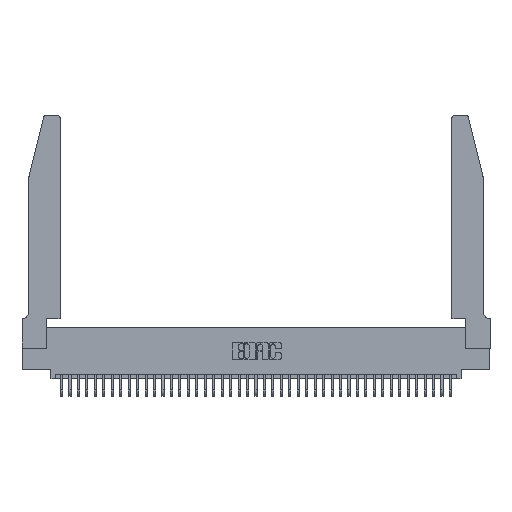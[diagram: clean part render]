
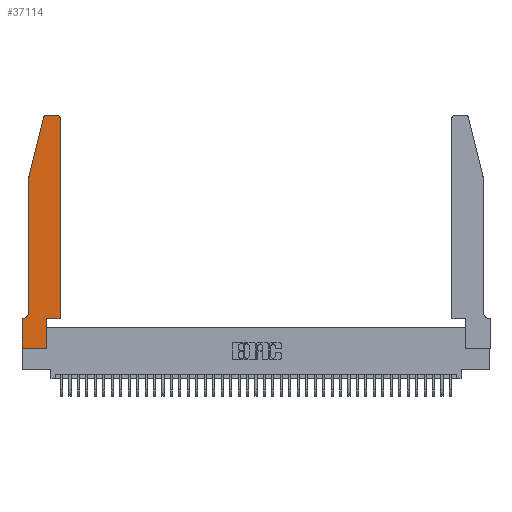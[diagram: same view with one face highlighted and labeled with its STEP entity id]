
A CAD part, top view. The second image highlights one B-rep face of the part: STEP entity #37114.
In plain terms, the highlighted planar face has unit normal (0, 0, 1).
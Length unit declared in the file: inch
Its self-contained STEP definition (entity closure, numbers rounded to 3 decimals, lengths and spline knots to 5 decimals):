
#99 = DIRECTION ( 'NONE',  ( 0., 0., -1. ) ) ;
#573 = VERTEX_POINT ( 'NONE', #23626 ) ;
#1099 = DIRECTION ( 'NONE',  ( -1., 0., 0. ) ) ;
#1113 = EDGE_CURVE ( 'NONE', #16538, #29028, #12907, .T. ) ;
#1559 = EDGE_CURVE ( 'NONE', #33392, #573, #23764, .T. ) ;
#1690 = VECTOR ( 'NONE', #23516, 39.37008 ) ;
#2515 = DIRECTION ( 'NONE',  ( 0., 1., 0. ) ) ;
#2747 = VERTEX_POINT ( 'NONE', #32198 ) ;
#3465 = EDGE_LOOP ( 'NONE', ( #12142, #10052, #17915, #38633, #32024, #14497, #37622, #26901, #16059, #22781, #12891, #10809 ) ) ;
#3533 = CARTESIAN_POINT ( 'NONE',  ( 0.2865, 0.35, 0.37 ) ) ;
#4565 = VECTOR ( 'NONE', #41761, 39.37008 ) ;
#4568 = DIRECTION ( 'NONE',  ( 0., 0., 1. ) ) ;
#5596 = AXIS2_PLACEMENT_3D ( 'NONE', #31060, #11277, #34377 ) ;
#6374 = EDGE_CURVE ( 'NONE', #573, #32763, #29571, .T. ) ;
#7736 = AXIS2_PLACEMENT_3D ( 'NONE', #20191, #99, #23435 ) ;
#7763 = CARTESIAN_POINT ( 'NONE',  ( 0.4205, 2.75, 0.37 ) ) ;
#8230 = EDGE_CURVE ( 'NONE', #33650, #16538, #13509, .T. ) ;
#8545 = DIRECTION ( 'NONE',  ( -0.239, -0.971, 0. ) ) ;
#9173 = CARTESIAN_POINT ( 'NONE',  ( 0.4505, 0.35, 0.37 ) ) ;
#9651 = EDGE_CURVE ( 'NONE', #21423, #33650, #29917, .T. ) ;
#10052 = ORIENTED_EDGE ( 'NONE', *, *, #20595, .T. ) ;
#10252 = CARTESIAN_POINT ( 'NONE',  ( 0.0755, 0.35, 0.37 ) ) ;
#10322 = LINE ( 'NONE', #9173, #26918 ) ;
#10646 = LINE ( 'NONE', #3533, #1690 ) ;
#10809 = ORIENTED_EDGE ( 'NONE', *, *, #21969, .T. ) ;
#10961 = VECTOR ( 'NONE', #20087, 39.37008 ) ;
#11277 = DIRECTION ( 'NONE',  ( 0., 0., 1. ) ) ;
#12142 = ORIENTED_EDGE ( 'NONE', *, *, #32826, .T. ) ;
#12891 = ORIENTED_EDGE ( 'NONE', *, *, #17405, .T. ) ;
#12907 = CIRCLE ( 'NONE', #7736, 0.07 ) ;
#13475 = CARTESIAN_POINT ( 'NONE',  ( 0., 0., 0.37 ) ) ;
#13509 = LINE ( 'NONE', #22235, #4565 ) ;
#14121 = CARTESIAN_POINT ( 'NONE',  ( 0., 0.35, 0.37 ) ) ;
#14497 = ORIENTED_EDGE ( 'NONE', *, *, #42621, .T. ) ;
#15692 = CIRCLE ( 'NONE', #16363, 0.03 ) ;
#16059 = ORIENTED_EDGE ( 'NONE', *, *, #39037, .T. ) ;
#16357 = VERTEX_POINT ( 'NONE', #7763 ) ;
#16363 = AXIS2_PLACEMENT_3D ( 'NONE', #18679, #41516, #21994 ) ;
#16538 = VERTEX_POINT ( 'NONE', #25025 ) ;
#16941 = LINE ( 'NONE', #37548, #32279 ) ;
#17405 = EDGE_CURVE ( 'NONE', #23726, #34346, #10322, .T. ) ;
#17824 = AXIS2_PLACEMENT_3D ( 'NONE', #24524, #4568, #27861 ) ;
#17915 = ORIENTED_EDGE ( 'NONE', *, *, #9651, .T. ) ;
#17928 = DIRECTION ( 'NONE',  ( 1., 0., 0. ) ) ;
#18191 = VECTOR ( 'NONE', #36628, 39.37008 ) ;
#18503 = CARTESIAN_POINT ( 'NONE',  ( 0.0755, 2., 0.37 ) ) ;
#18679 = CARTESIAN_POINT ( 'NONE',  ( 0.4205, 2.72, 0.37 ) ) ;
#19126 = CARTESIAN_POINT ( 'NONE',  ( 0., 0., 0.37 ) ) ;
#19732 = LINE ( 'NONE', #21181, #37126 ) ;
#19895 = EDGE_CURVE ( 'NONE', #27673, #23726, #16941, .T. ) ;
#20046 = CARTESIAN_POINT ( 'NONE',  ( 0.0055, 0.35, 0.37 ) ) ;
#20087 = DIRECTION ( 'NONE',  ( 1., 0., 0. ) ) ;
#20191 = CARTESIAN_POINT ( 'NONE',  ( 0.0055, 0.42, 0.37 ) ) ;
#20595 = EDGE_CURVE ( 'NONE', #2747, #21423, #40945, .T. ) ;
#21181 = CARTESIAN_POINT ( 'NONE',  ( 0.2605, 2.75, 0.37 ) ) ;
#21423 = VERTEX_POINT ( 'NONE', #29025 ) ;
#21969 = EDGE_CURVE ( 'NONE', #34346, #16357, #15692, .T. ) ;
#21994 = DIRECTION ( 'NONE',  ( 1., 0., 0. ) ) ;
#22235 = CARTESIAN_POINT ( 'NONE',  ( 0.0755, 2., 0.37 ) ) ;
#22482 = CARTESIAN_POINT ( 'NONE',  ( 0.4505, 2.72, 0.37 ) ) ;
#22781 = ORIENTED_EDGE ( 'NONE', *, *, #19895, .T. ) ;
#23435 = DIRECTION ( 'NONE',  ( -1., 0., 0. ) ) ;
#23516 = DIRECTION ( 'NONE',  ( 0., 1., 0. ) ) ;
#23626 = CARTESIAN_POINT ( 'NONE',  ( 0., 0., 0.37 ) ) ;
#23726 = VERTEX_POINT ( 'NONE', #32358 ) ;
#23764 = LINE ( 'NONE', #19126, #32511 ) ;
#24264 = VECTOR ( 'NONE', #8545, 39.37008 ) ;
#24524 = CARTESIAN_POINT ( 'NONE',  ( 0., 0.35, 0.37 ) ) ;
#25025 = CARTESIAN_POINT ( 'NONE',  ( 0.0755, 0.42, 0.37 ) ) ;
#26901 = ORIENTED_EDGE ( 'NONE', *, *, #6374, .T. ) ;
#26918 = VECTOR ( 'NONE', #2515, 39.37008 ) ;
#27673 = VERTEX_POINT ( 'NONE', #32595 ) ;
#27861 = DIRECTION ( 'NONE',  ( 1., 0., 0. ) ) ;
#27943 = LINE ( 'NONE', #10252, #18191 ) ;
#28531 = CARTESIAN_POINT ( 'NONE',  ( 0.0755, 2., 0.37 ) ) ;
#29025 = CARTESIAN_POINT ( 'NONE',  ( 0.25487, 2.72718, 0.37 ) ) ;
#29028 = VERTEX_POINT ( 'NONE', #20046 ) ;
#29571 = LINE ( 'NONE', #13475, #10961 ) ;
#29917 = LINE ( 'NONE', #28531, #24264 ) ;
#30744 = CARTESIAN_POINT ( 'NONE',  ( 0.2865, 0., 0.37 ) ) ;
#31060 = CARTESIAN_POINT ( 'NONE',  ( 0.284, 2.72, 0.37 ) ) ;
#32024 = ORIENTED_EDGE ( 'NONE', *, *, #1113, .T. ) ;
#32198 = CARTESIAN_POINT ( 'NONE',  ( 0.284, 2.75, 0.37 ) ) ;
#32279 = VECTOR ( 'NONE', #17928, 39.37008 ) ;
#32358 = CARTESIAN_POINT ( 'NONE',  ( 0.4505, 0.35, 0.37 ) ) ;
#32511 = VECTOR ( 'NONE', #41945, 39.37008 ) ;
#32595 = CARTESIAN_POINT ( 'NONE',  ( 0.2865, 0.35, 0.37 ) ) ;
#32763 = VERTEX_POINT ( 'NONE', #30744 ) ;
#32826 = EDGE_CURVE ( 'NONE', #16357, #2747, #19732, .T. ) ;
#33392 = VERTEX_POINT ( 'NONE', #14121 ) ;
#33650 = VERTEX_POINT ( 'NONE', #18503 ) ;
#34346 = VERTEX_POINT ( 'NONE', #22482 ) ;
#34377 = DIRECTION ( 'NONE',  ( 1., 0., 0. ) ) ;
#36628 = DIRECTION ( 'NONE',  ( -1., 0., 0. ) ) ;
#37114 = ADVANCED_FACE ( 'NONE', ( #41209 ), #40832, .T. ) ;
#37126 = VECTOR ( 'NONE', #1099, 39.37008 ) ;
#37548 = CARTESIAN_POINT ( 'NONE',  ( 0.4505, 0.35, 0.37 ) ) ;
#37622 = ORIENTED_EDGE ( 'NONE', *, *, #1559, .T. ) ;
#38633 = ORIENTED_EDGE ( 'NONE', *, *, #8230, .T. ) ;
#39037 = EDGE_CURVE ( 'NONE', #32763, #27673, #10646, .T. ) ;
#40832 = PLANE ( 'NONE',  #17824 ) ;
#40945 = CIRCLE ( 'NONE', #5596, 0.03 ) ;
#41209 = FACE_OUTER_BOUND ( 'NONE', #3465, .T. ) ;
#41516 = DIRECTION ( 'NONE',  ( 0., 0., 1. ) ) ;
#41761 = DIRECTION ( 'NONE',  ( 0., -1., 0. ) ) ;
#41945 = DIRECTION ( 'NONE',  ( 0., -1., 0. ) ) ;
#42621 = EDGE_CURVE ( 'NONE', #29028, #33392, #27943, .T. ) ;
